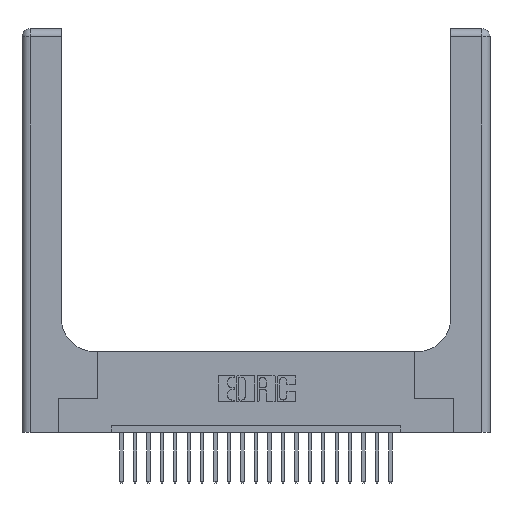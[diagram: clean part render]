
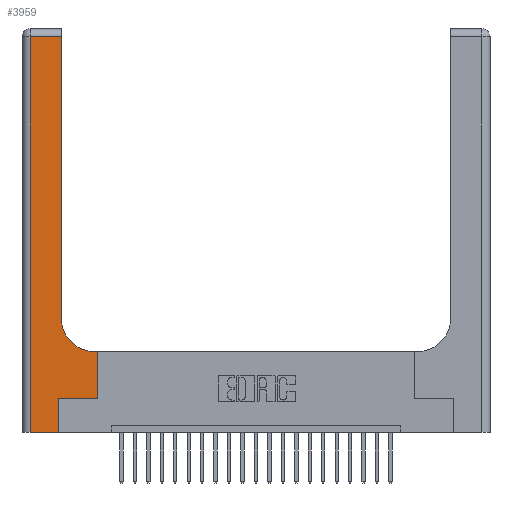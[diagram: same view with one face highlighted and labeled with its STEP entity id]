
A CAD part, top view. The second image highlights one B-rep face of the part: STEP entity #3959.
In plain terms, the highlighted planar face has unit normal (0, 0, 1).
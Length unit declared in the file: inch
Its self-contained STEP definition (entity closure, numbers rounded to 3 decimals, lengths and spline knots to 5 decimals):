
#131 = DIRECTION ( 'NONE',  ( -1., 0., 0. ) ) ;
#156 = DIRECTION ( 'NONE',  ( 0., 1., 0. ) ) ;
#184 = DIRECTION ( 'NONE',  ( 0., 0., -1. ) ) ;
#655 = DIRECTION ( 'NONE',  ( 1., 0., 0. ) ) ;
#758 = CARTESIAN_POINT ( 'NONE',  ( 0.5585, 0.25, 0.37 ) ) ;
#1089 = VERTEX_POINT ( 'NONE', #4412 ) ;
#1738 = EDGE_CURVE ( 'NONE', #4621, #13950, #14981, .T. ) ;
#1870 = VERTEX_POINT ( 'NONE', #16743 ) ;
#2012 = VECTOR ( 'NONE', #19492, 39.37008 ) ;
#2411 = CIRCLE ( 'NONE', #5283, 0.25 ) ;
#2553 = ORIENTED_EDGE ( 'NONE', *, *, #13369, .T. ) ;
#2706 = EDGE_CURVE ( 'NONE', #22556, #1089, #17276, .T. ) ;
#3871 = LINE ( 'NONE', #16998, #12733 ) ;
#3959 = ADVANCED_FACE ( 'NONE', ( #21503 ), #13481, .F. ) ;
#4412 = CARTESIAN_POINT ( 'NONE',  ( 0.5585, 0.6, 0.37 ) ) ;
#4539 = EDGE_CURVE ( 'NONE', #13950, #12095, #16645, .T. ) ;
#4621 = VERTEX_POINT ( 'NONE', #10179 ) ;
#5256 = CARTESIAN_POINT ( 'NONE',  ( 0.269, 0.25, 0.37 ) ) ;
#5283 = AXIS2_PLACEMENT_3D ( 'NONE', #20460, #184, #11130 ) ;
#5354 = CARTESIAN_POINT ( 'NONE',  ( 0.5415, 0.6, 0.37 ) ) ;
#5631 = VECTOR ( 'NONE', #655, 39.37008 ) ;
#5663 = VERTEX_POINT ( 'NONE', #23741 ) ;
#5727 = DIRECTION ( 'NONE',  ( 1., 0., 0. ) ) ;
#5757 = CARTESIAN_POINT ( 'NONE',  ( 0.06, 2.94, 0.37 ) ) ;
#6581 = CARTESIAN_POINT ( 'NONE',  ( 0., 2.94, 0.37 ) ) ;
#7456 = LINE ( 'NONE', #16818, #18966 ) ;
#8013 = DIRECTION ( 'NONE',  ( -1., 0., 0. ) ) ;
#9937 = VECTOR ( 'NONE', #11858, 39.37008 ) ;
#10179 = CARTESIAN_POINT ( 'NONE',  ( 0.2915, 2.94, 0.37 ) ) ;
#10761 = VECTOR ( 'NONE', #5727, 39.37008 ) ;
#10983 = EDGE_CURVE ( 'NONE', #12095, #5663, #15722, .T. ) ;
#11043 = VERTEX_POINT ( 'NONE', #5354 ) ;
#11130 = DIRECTION ( 'NONE',  ( 1., 0., 0. ) ) ;
#11158 = ORIENTED_EDGE ( 'NONE', *, *, #10983, .T. ) ;
#11556 = DIRECTION ( 'NONE',  ( -1., 0., 0. ) ) ;
#11858 = DIRECTION ( 'NONE',  ( 0., 1., 0. ) ) ;
#11888 = CARTESIAN_POINT ( 'NONE',  ( 0., 3., 0.37 ) ) ;
#12095 = VERTEX_POINT ( 'NONE', #14403 ) ;
#12733 = VECTOR ( 'NONE', #156, 39.37008 ) ;
#13287 = EDGE_CURVE ( 'NONE', #20023, #22556, #15679, .T. ) ;
#13319 = DIRECTION ( 'NONE',  ( 0., 0., -1. ) ) ;
#13369 = EDGE_CURVE ( 'NONE', #1870, #4621, #3871, .T. ) ;
#13481 = PLANE ( 'NONE',  #13817 ) ;
#13588 = CARTESIAN_POINT ( 'NONE',  ( 0.06, 3., 0.37 ) ) ;
#13817 = AXIS2_PLACEMENT_3D ( 'NONE', #11888, #13319, #11556 ) ;
#13931 = CARTESIAN_POINT ( 'NONE',  ( 0., 0., 0.37 ) ) ;
#13950 = VERTEX_POINT ( 'NONE', #5757 ) ;
#14403 = CARTESIAN_POINT ( 'NONE',  ( 0.06, 0., 0.37 ) ) ;
#14817 = EDGE_CURVE ( 'NONE', #1089, #11043, #7456, .T. ) ;
#14874 = LINE ( 'NONE', #23025, #9937 ) ;
#14981 = LINE ( 'NONE', #6581, #17900 ) ;
#15042 = ORIENTED_EDGE ( 'NONE', *, *, #1738, .T. ) ;
#15149 = VECTOR ( 'NONE', #20997, 39.37008 ) ;
#15679 = LINE ( 'NONE', #18533, #10761 ) ;
#15722 = LINE ( 'NONE', #13931, #5631 ) ;
#16010 = EDGE_CURVE ( 'NONE', #5663, #20023, #14874, .T. ) ;
#16549 = ORIENTED_EDGE ( 'NONE', *, *, #2706, .T. ) ;
#16645 = LINE ( 'NONE', #13588, #15149 ) ;
#16743 = CARTESIAN_POINT ( 'NONE',  ( 0.2915, 0.85, 0.37 ) ) ;
#16818 = CARTESIAN_POINT ( 'NONE',  ( 0.2915, 0.6, 0.37 ) ) ;
#16998 = CARTESIAN_POINT ( 'NONE',  ( 0.2915, 3., 0.37 ) ) ;
#17276 = LINE ( 'NONE', #23034, #2012 ) ;
#17473 = EDGE_CURVE ( 'NONE', #11043, #1870, #2411, .T. ) ;
#17900 = VECTOR ( 'NONE', #8013, 39.37008 ) ;
#18533 = CARTESIAN_POINT ( 'NONE',  ( 0.269, 0.25, 0.37 ) ) ;
#18966 = VECTOR ( 'NONE', #131, 39.37008 ) ;
#19336 = EDGE_LOOP ( 'NONE', ( #2553, #15042, #20523, #11158, #23006, #22945, #16549, #20068, #20605 ) ) ;
#19492 = DIRECTION ( 'NONE',  ( 0., 1., 0. ) ) ;
#20023 = VERTEX_POINT ( 'NONE', #5256 ) ;
#20068 = ORIENTED_EDGE ( 'NONE', *, *, #14817, .T. ) ;
#20460 = CARTESIAN_POINT ( 'NONE',  ( 0.5415, 0.85, 0.37 ) ) ;
#20523 = ORIENTED_EDGE ( 'NONE', *, *, #4539, .T. ) ;
#20605 = ORIENTED_EDGE ( 'NONE', *, *, #17473, .T. ) ;
#20997 = DIRECTION ( 'NONE',  ( 0., -1., 0. ) ) ;
#21503 = FACE_OUTER_BOUND ( 'NONE', #19336, .T. ) ;
#22556 = VERTEX_POINT ( 'NONE', #758 ) ;
#22945 = ORIENTED_EDGE ( 'NONE', *, *, #13287, .T. ) ;
#23006 = ORIENTED_EDGE ( 'NONE', *, *, #16010, .T. ) ;
#23025 = CARTESIAN_POINT ( 'NONE',  ( 0.269, 0., 0.37 ) ) ;
#23034 = CARTESIAN_POINT ( 'NONE',  ( 0.5585, 0.25, 0.37 ) ) ;
#23741 = CARTESIAN_POINT ( 'NONE',  ( 0.269, 0., 0.37 ) ) ;
